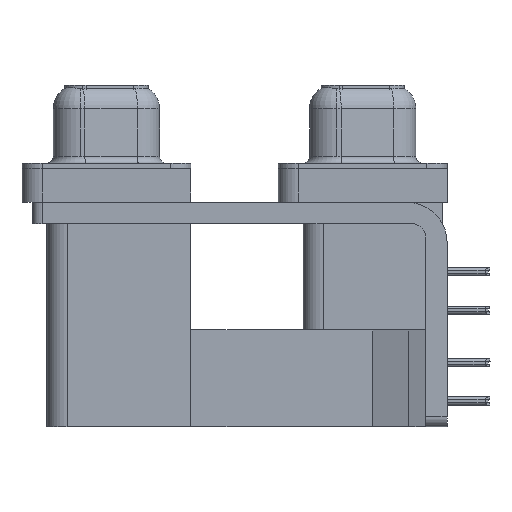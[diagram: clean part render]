
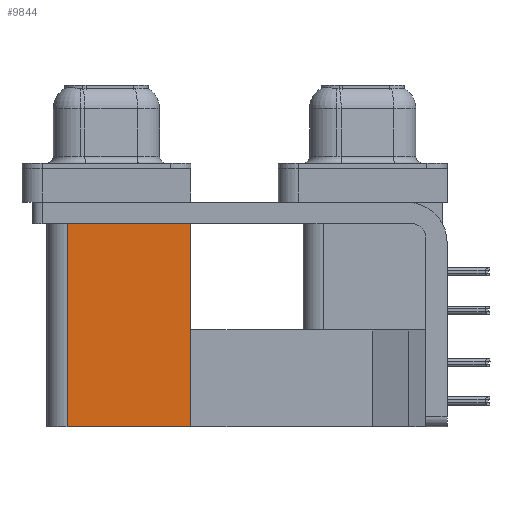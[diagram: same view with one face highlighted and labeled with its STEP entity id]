
A CAD part, left-side view. The second image highlights one B-rep face of the part: STEP entity #9844.
In plain terms, the highlighted planar face has unit normal (-1, 0, 0).
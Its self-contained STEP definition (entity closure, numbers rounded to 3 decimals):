
#585 = AXIS2_PLACEMENT_3D ( 'NONE', #32499, #20281, #10889 ) ;
#2255 = FACE_OUTER_BOUND ( 'NONE', #8852, .T. ) ;
#2810 = DIRECTION ( 'NONE',  ( 0., 1., 0. ) ) ;
#4261 = CARTESIAN_POINT ( 'NONE',  ( 3.79, 12.775, -19.2 ) ) ;
#4836 = EDGE_CURVE ( 'NONE', #35915, #17162, #36847, .T. ) ;
#8326 = CARTESIAN_POINT ( 'NONE',  ( 3.79, 21.975, -19.2 ) ) ;
#8477 = VECTOR ( 'NONE', #22911, 1000. ) ;
#8852 = EDGE_LOOP ( 'NONE', ( #38243, #31570, #12841, #34620 ) ) ;
#9734 = VECTOR ( 'NONE', #34412, 1000. ) ;
#9844 = ADVANCED_FACE ( 'NONE', ( #2255 ), #20083, .F. ) ;
#10731 = CARTESIAN_POINT ( 'NONE',  ( 3.79, 21.975, -19.2 ) ) ;
#10889 = DIRECTION ( 'NONE',  ( 0., 1., 0. ) ) ;
#12841 = ORIENTED_EDGE ( 'NONE', *, *, #4836, .F. ) ;
#14055 = EDGE_CURVE ( 'NONE', #17162, #37174, #35557, .T. ) ;
#17162 = VERTEX_POINT ( 'NONE', #8326 ) ;
#18786 = CARTESIAN_POINT ( 'NONE',  ( 3.79, 12.775, -19.2 ) ) ;
#19080 = VECTOR ( 'NONE', #2810, 1000. ) ;
#19931 = CARTESIAN_POINT ( 'NONE',  ( 3.79, 21.975, -2.5 ) ) ;
#20083 = PLANE ( 'NONE',  #585 ) ;
#20281 = DIRECTION ( 'NONE',  ( 1., 0., 0. ) ) ;
#20696 = CARTESIAN_POINT ( 'NONE',  ( 3.79, 12.775, -2.5 ) ) ;
#22911 = DIRECTION ( 'NONE',  ( 0., 0., 1. ) ) ;
#24645 = CARTESIAN_POINT ( 'NONE',  ( 3.79, 12.775, -19.2 ) ) ;
#26168 = EDGE_CURVE ( 'NONE', #35915, #38909, #30855, .T. ) ;
#30162 = VECTOR ( 'NONE', #37469, 1000. ) ;
#30847 = CARTESIAN_POINT ( 'NONE',  ( 3.79, 12.775, -2.5 ) ) ;
#30855 = LINE ( 'NONE', #24645, #30162 ) ;
#31570 = ORIENTED_EDGE ( 'NONE', *, *, #14055, .F. ) ;
#32499 = CARTESIAN_POINT ( 'NONE',  ( 3.79, 12.775, -19.2 ) ) ;
#34412 = DIRECTION ( 'NONE',  ( 0., 1., 0. ) ) ;
#34620 = ORIENTED_EDGE ( 'NONE', *, *, #26168, .T. ) ;
#35557 = LINE ( 'NONE', #10731, #8477 ) ;
#35915 = VERTEX_POINT ( 'NONE', #4261 ) ;
#36473 = LINE ( 'NONE', #30847, #19080 ) ;
#36847 = LINE ( 'NONE', #18786, #9734 ) ;
#37174 = VERTEX_POINT ( 'NONE', #19931 ) ;
#37469 = DIRECTION ( 'NONE',  ( 0., 0., 1. ) ) ;
#38243 = ORIENTED_EDGE ( 'NONE', *, *, #39580, .T. ) ;
#38909 = VERTEX_POINT ( 'NONE', #20696 ) ;
#39580 = EDGE_CURVE ( 'NONE', #38909, #37174, #36473, .T. ) ;
